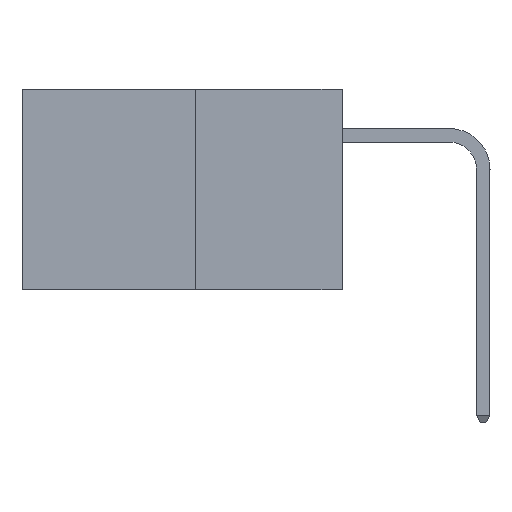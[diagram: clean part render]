
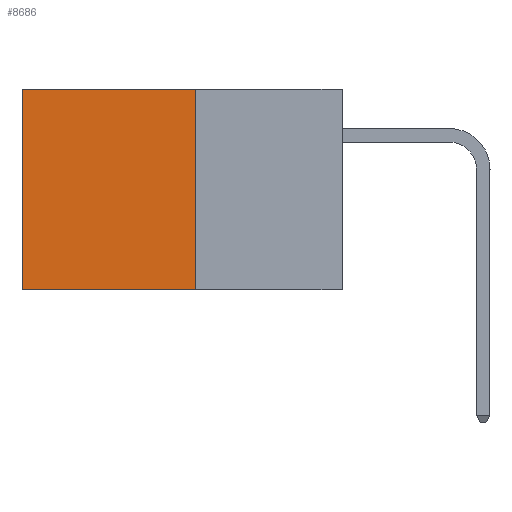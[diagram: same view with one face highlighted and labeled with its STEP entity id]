
A CAD part, left-side view. The second image highlights one B-rep face of the part: STEP entity #8686.
In plain terms, the highlighted planar face has unit normal (-1, 0, 0).
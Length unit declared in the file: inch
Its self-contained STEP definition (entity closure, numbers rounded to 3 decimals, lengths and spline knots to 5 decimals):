
#1167 = DIRECTION ( 'NONE',  ( 0., 1., 0. ) ) ;
#2087 = EDGE_CURVE ( 'NONE', #4828, #26959, #16238, .T. ) ;
#2286 = VECTOR ( 'NONE', #19581, 39.37008 ) ;
#3846 = CARTESIAN_POINT ( 'NONE',  ( 0.277, 0.27, -0.37 ) ) ;
#4828 = VERTEX_POINT ( 'NONE', #16234 ) ;
#6097 = ORIENTED_EDGE ( 'NONE', *, *, #2087, .F. ) ;
#6171 = LINE ( 'NONE', #22131, #19167 ) ;
#8686 = ADVANCED_FACE ( 'NONE', ( #26260 ), #23228, .F. ) ;
#9647 = VERTEX_POINT ( 'NONE', #14072 ) ;
#11630 = EDGE_LOOP ( 'NONE', ( #31102, #16265, #6097, #19076 ) ) ;
#12462 = CARTESIAN_POINT ( 'NONE',  ( 0.277, 0.59, -0.37 ) ) ;
#12565 = LINE ( 'NONE', #24356, #32536 ) ;
#14065 = DIRECTION ( 'NONE',  ( 0., 1., 0. ) ) ;
#14072 = CARTESIAN_POINT ( 'NONE',  ( 0.277, 0.59, 0. ) ) ;
#14224 = AXIS2_PLACEMENT_3D ( 'NONE', #3846, #25089, #24579 ) ;
#16234 = CARTESIAN_POINT ( 'NONE',  ( 0.277, 0.27, 0. ) ) ;
#16238 = LINE ( 'NONE', #20321, #2286 ) ;
#16265 = ORIENTED_EDGE ( 'NONE', *, *, #29570, .F. ) ;
#17454 = VECTOR ( 'NONE', #19934, 39.37008 ) ;
#19076 = ORIENTED_EDGE ( 'NONE', *, *, #33432, .T. ) ;
#19167 = VECTOR ( 'NONE', #1167, 39.37008 ) ;
#19581 = DIRECTION ( 'NONE',  ( 0., 0., -1. ) ) ;
#19828 = CARTESIAN_POINT ( 'NONE',  ( 0.277, 0.59, -0.37 ) ) ;
#19934 = DIRECTION ( 'NONE',  ( 0., 0., -1. ) ) ;
#20321 = CARTESIAN_POINT ( 'NONE',  ( 0.277, 0.27, -0.37 ) ) ;
#22131 = CARTESIAN_POINT ( 'NONE',  ( 0.277, 0.27, 0. ) ) ;
#23228 = PLANE ( 'NONE',  #14224 ) ;
#24356 = CARTESIAN_POINT ( 'NONE',  ( 0.277, 0.27, -0.37 ) ) ;
#24579 = DIRECTION ( 'NONE',  ( 0., 0., -1. ) ) ;
#25089 = DIRECTION ( 'NONE',  ( 1., 0., 0. ) ) ;
#26260 = FACE_OUTER_BOUND ( 'NONE', #11630, .T. ) ;
#26851 = EDGE_CURVE ( 'NONE', #9647, #32182, #31328, .T. ) ;
#26959 = VERTEX_POINT ( 'NONE', #33337 ) ;
#29570 = EDGE_CURVE ( 'NONE', #26959, #32182, #12565, .T. ) ;
#31102 = ORIENTED_EDGE ( 'NONE', *, *, #26851, .T. ) ;
#31328 = LINE ( 'NONE', #19828, #17454 ) ;
#32182 = VERTEX_POINT ( 'NONE', #12462 ) ;
#32536 = VECTOR ( 'NONE', #14065, 39.37008 ) ;
#33337 = CARTESIAN_POINT ( 'NONE',  ( 0.277, 0.27, -0.37 ) ) ;
#33432 = EDGE_CURVE ( 'NONE', #4828, #9647, #6171, .T. ) ;
